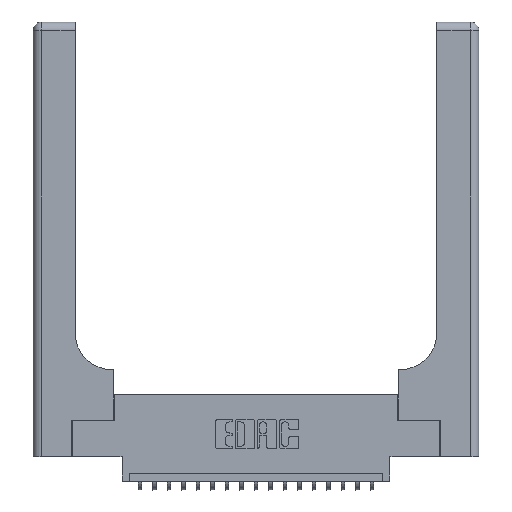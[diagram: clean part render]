
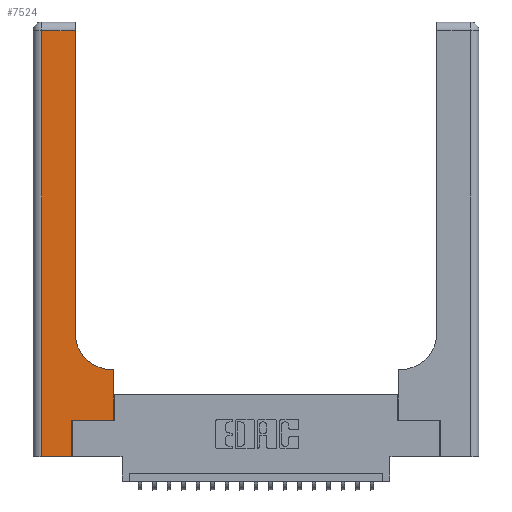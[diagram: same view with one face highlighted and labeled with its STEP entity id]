
A CAD part, top view. The second image highlights one B-rep face of the part: STEP entity #7524.
In plain terms, the highlighted planar face has unit normal (0, 0, 1).
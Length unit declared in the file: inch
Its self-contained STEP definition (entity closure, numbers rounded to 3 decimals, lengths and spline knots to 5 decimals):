
#220 = DIRECTION ( 'NONE',  ( 0., -1., 0. ) ) ;
#226 = LINE ( 'NONE', #17265, #9848 ) ;
#235 = DIRECTION ( 'NONE',  ( 1., 0., 0. ) ) ;
#382 = DIRECTION ( 'NONE',  ( 0., 1., 0. ) ) ;
#804 = VERTEX_POINT ( 'NONE', #15550 ) ;
#973 = ORIENTED_EDGE ( 'NONE', *, *, #11468, .T. ) ;
#1176 = VECTOR ( 'NONE', #13912, 39.37008 ) ;
#1743 = CARTESIAN_POINT ( 'NONE',  ( 0.06, 3., 0.37 ) ) ;
#2100 = ORIENTED_EDGE ( 'NONE', *, *, #2197, .T. ) ;
#2197 = EDGE_CURVE ( 'NONE', #4234, #5703, #18289, .T. ) ;
#2354 = EDGE_CURVE ( 'NONE', #15965, #14164, #15927, .T. ) ;
#3510 = LINE ( 'NONE', #1743, #11525 ) ;
#3625 = VERTEX_POINT ( 'NONE', #14225 ) ;
#3737 = LINE ( 'NONE', #10130, #17218 ) ;
#4234 = VERTEX_POINT ( 'NONE', #4432 ) ;
#4275 = LINE ( 'NONE', #6761, #15229 ) ;
#4432 = CARTESIAN_POINT ( 'NONE',  ( 0.269, 0.25, 0.37 ) ) ;
#4639 = DIRECTION ( 'NONE',  ( 1., 0., 0. ) ) ;
#5034 = DIRECTION ( 'NONE',  ( -1., 0., 0. ) ) ;
#5056 = VERTEX_POINT ( 'NONE', #21569 ) ;
#5347 = CARTESIAN_POINT ( 'NONE',  ( 0.269, 0., 0.37 ) ) ;
#5703 = VERTEX_POINT ( 'NONE', #5802 ) ;
#5802 = CARTESIAN_POINT ( 'NONE',  ( 0.5585, 0.25, 0.37 ) ) ;
#6105 = LINE ( 'NONE', #5347, #6377 ) ;
#6329 = AXIS2_PLACEMENT_3D ( 'NONE', #7448, #19145, #4639 ) ;
#6377 = VECTOR ( 'NONE', #382, 39.37008 ) ;
#6465 = DIRECTION ( 'NONE',  ( 0., 1., 0. ) ) ;
#6761 = CARTESIAN_POINT ( 'NONE',  ( 0.2915, 3., 0.37 ) ) ;
#7096 = ORIENTED_EDGE ( 'NONE', *, *, #16781, .T. ) ;
#7305 = DIRECTION ( 'NONE',  ( -1., 0., 0. ) ) ;
#7347 = CARTESIAN_POINT ( 'NONE',  ( 0.2915, 0.85, 0.37 ) ) ;
#7400 = LINE ( 'NONE', #20646, #1176 ) ;
#7448 = CARTESIAN_POINT ( 'NONE',  ( 0.5415, 0.85, 0.37 ) ) ;
#7524 = ADVANCED_FACE ( 'NONE', ( #11141 ), #10580, .F. ) ;
#7783 = EDGE_CURVE ( 'NONE', #3625, #5056, #226, .T. ) ;
#8575 = ORIENTED_EDGE ( 'NONE', *, *, #15214, .T. ) ;
#9439 = CARTESIAN_POINT ( 'NONE',  ( 0.269, 0., 0.37 ) ) ;
#9539 = DIRECTION ( 'NONE',  ( 1., 0., 0. ) ) ;
#9848 = VECTOR ( 'NONE', #7305, 39.37008 ) ;
#10130 = CARTESIAN_POINT ( 'NONE',  ( 0., 0., 0.37 ) ) ;
#10321 = EDGE_CURVE ( 'NONE', #5703, #804, #7400, .T. ) ;
#10580 = PLANE ( 'NONE',  #13216 ) ;
#11094 = VERTEX_POINT ( 'NONE', #9439 ) ;
#11141 = FACE_OUTER_BOUND ( 'NONE', #19602, .T. ) ;
#11468 = EDGE_CURVE ( 'NONE', #5056, #13224, #3510, .T. ) ;
#11525 = VECTOR ( 'NONE', #220, 39.37008 ) ;
#12168 = CARTESIAN_POINT ( 'NONE',  ( 0., 3., 0.37 ) ) ;
#12183 = ORIENTED_EDGE ( 'NONE', *, *, #12275, .T. ) ;
#12275 = EDGE_CURVE ( 'NONE', #13224, #11094, #3737, .T. ) ;
#12301 = DIRECTION ( 'NONE',  ( 0., 0., -1. ) ) ;
#13216 = AXIS2_PLACEMENT_3D ( 'NONE', #12168, #12301, #20601 ) ;
#13224 = VERTEX_POINT ( 'NONE', #21568 ) ;
#13370 = CARTESIAN_POINT ( 'NONE',  ( 0.2915, 0.6, 0.37 ) ) ;
#13912 = DIRECTION ( 'NONE',  ( 0., 1., 0. ) ) ;
#14164 = VERTEX_POINT ( 'NONE', #7347 ) ;
#14225 = CARTESIAN_POINT ( 'NONE',  ( 0.2915, 2.94, 0.37 ) ) ;
#14409 = VECTOR ( 'NONE', #9539, 39.37008 ) ;
#14512 = VECTOR ( 'NONE', #5034, 39.37008 ) ;
#15214 = EDGE_CURVE ( 'NONE', #804, #15965, #18668, .T. ) ;
#15229 = VECTOR ( 'NONE', #6465, 39.37008 ) ;
#15550 = CARTESIAN_POINT ( 'NONE',  ( 0.5585, 0.6, 0.37 ) ) ;
#15927 = CIRCLE ( 'NONE', #6329, 0.25 ) ;
#15965 = VERTEX_POINT ( 'NONE', #20036 ) ;
#16221 = CARTESIAN_POINT ( 'NONE',  ( 0.269, 0.25, 0.37 ) ) ;
#16425 = EDGE_CURVE ( 'NONE', #11094, #4234, #6105, .T. ) ;
#16781 = EDGE_CURVE ( 'NONE', #14164, #3625, #4275, .T. ) ;
#16980 = ORIENTED_EDGE ( 'NONE', *, *, #10321, .T. ) ;
#17218 = VECTOR ( 'NONE', #235, 39.37008 ) ;
#17265 = CARTESIAN_POINT ( 'NONE',  ( 0., 2.94, 0.37 ) ) ;
#17462 = ORIENTED_EDGE ( 'NONE', *, *, #2354, .T. ) ;
#18289 = LINE ( 'NONE', #16221, #14409 ) ;
#18668 = LINE ( 'NONE', #13370, #14512 ) ;
#19145 = DIRECTION ( 'NONE',  ( 0., 0., -1. ) ) ;
#19602 = EDGE_LOOP ( 'NONE', ( #7096, #21030, #973, #12183, #19759, #2100, #16980, #8575, #17462 ) ) ;
#19759 = ORIENTED_EDGE ( 'NONE', *, *, #16425, .T. ) ;
#20036 = CARTESIAN_POINT ( 'NONE',  ( 0.5415, 0.6, 0.37 ) ) ;
#20601 = DIRECTION ( 'NONE',  ( -1., 0., 0. ) ) ;
#20646 = CARTESIAN_POINT ( 'NONE',  ( 0.5585, 0.25, 0.37 ) ) ;
#21030 = ORIENTED_EDGE ( 'NONE', *, *, #7783, .T. ) ;
#21568 = CARTESIAN_POINT ( 'NONE',  ( 0.06, 0., 0.37 ) ) ;
#21569 = CARTESIAN_POINT ( 'NONE',  ( 0.06, 2.94, 0.37 ) ) ;
